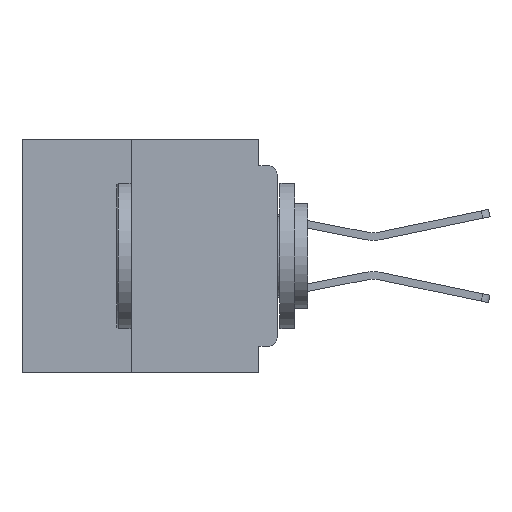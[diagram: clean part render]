
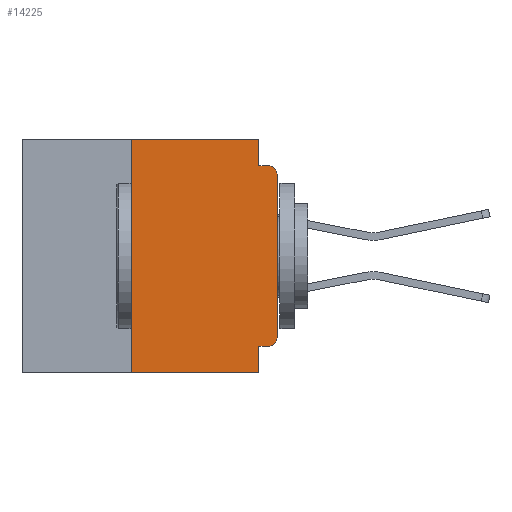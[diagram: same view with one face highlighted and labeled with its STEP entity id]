
A CAD part, left-side view. The second image highlights one B-rep face of the part: STEP entity #14225.
In plain terms, the highlighted planar face has unit normal (-1, 0, 0).
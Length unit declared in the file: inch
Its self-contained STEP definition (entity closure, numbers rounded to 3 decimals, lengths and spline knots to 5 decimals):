
#232 = CARTESIAN_POINT ( 'NONE',  ( 0., 0.25, 0. ) ) ;
#1483 = CARTESIAN_POINT ( 'NONE',  ( 0., 0.031, 0. ) ) ;
#1991 = DIRECTION ( 'NONE',  ( 0., 0., -1. ) ) ;
#2050 = VECTOR ( 'NONE', #49819, 39.37008 ) ;
#2190 = VERTEX_POINT ( 'NONE', #29514 ) ;
#3224 = DIRECTION ( 'NONE',  ( 0., 0., 1. ) ) ;
#3545 = LINE ( 'NONE', #34313, #13835 ) ;
#3659 = EDGE_CURVE ( 'NONE', #49063, #10505, #14028, .T. ) ;
#4939 = EDGE_CURVE ( 'NONE', #13202, #49063, #8471, .T. ) ;
#6959 = DIRECTION ( 'NONE',  ( 0., -1., 0. ) ) ;
#7059 = ORIENTED_EDGE ( 'NONE', *, *, #27937, .F. ) ;
#7067 = AXIS2_PLACEMENT_3D ( 'NONE', #41089, #18066, #44920 ) ;
#7124 = CARTESIAN_POINT ( 'NONE',  ( 0., 0.25, -0.4 ) ) ;
#7233 = CARTESIAN_POINT ( 'NONE',  ( 0., 0., -0.06 ) ) ;
#8471 = LINE ( 'NONE', #38049, #17540 ) ;
#8766 = LINE ( 'NONE', #43683, #28093 ) ;
#8858 = FACE_OUTER_BOUND ( 'NONE', #10433, .T. ) ;
#9204 = VERTEX_POINT ( 'NONE', #7233 ) ;
#9404 = EDGE_CURVE ( 'NONE', #9204, #26934, #10575, .T. ) ;
#10433 = EDGE_LOOP ( 'NONE', ( #49125, #35379, #38479, #33665, #41463, #27238, #47545, #17439, #7059, #19909 ) ) ;
#10505 = VERTEX_POINT ( 'NONE', #47153 ) ;
#10575 = CIRCLE ( 'NONE', #38469, 0.015 ) ;
#13202 = VERTEX_POINT ( 'NONE', #232 ) ;
#13835 = VECTOR ( 'NONE', #49495, 39.37008 ) ;
#14028 = LINE ( 'NONE', #1483, #23120 ) ;
#14183 = PLANE ( 'NONE',  #7067 ) ;
#14225 = ADVANCED_FACE ( 'NONE', ( #8858 ), #14183, .F. ) ;
#15724 = CARTESIAN_POINT ( 'NONE',  ( 0., 0.015, -0.34 ) ) ;
#16689 = CARTESIAN_POINT ( 'NONE',  ( 0., 0.25, -0.4 ) ) ;
#17439 = ORIENTED_EDGE ( 'NONE', *, *, #18331, .F. ) ;
#17540 = VECTOR ( 'NONE', #34218, 39.37008 ) ;
#18066 = DIRECTION ( 'NONE',  ( 1., 0., 0. ) ) ;
#18331 = EDGE_CURVE ( 'NONE', #26631, #31241, #3545, .T. ) ;
#18851 = CARTESIAN_POINT ( 'NONE',  ( 0., 0., -0.045 ) ) ;
#19579 = AXIS2_PLACEMENT_3D ( 'NONE', #15724, #42595, #19598 ) ;
#19598 = DIRECTION ( 'NONE',  ( 0., 0., -1. ) ) ;
#19909 = ORIENTED_EDGE ( 'NONE', *, *, #20971, .T. ) ;
#19921 = DIRECTION ( 'NONE',  ( -1., 0., 0. ) ) ;
#20550 = DIRECTION ( 'NONE',  ( 0., 0., 1. ) ) ;
#20561 = LINE ( 'NONE', #18851, #40963 ) ;
#20971 = EDGE_CURVE ( 'NONE', #44057, #2190, #44777, .T. ) ;
#21524 = VECTOR ( 'NONE', #6959, 39.37008 ) ;
#22809 = CARTESIAN_POINT ( 'NONE',  ( 0., 0.015, -0.045 ) ) ;
#23120 = VECTOR ( 'NONE', #1991, 39.37008 ) ;
#23303 = EDGE_CURVE ( 'NONE', #10505, #26934, #20561, .T. ) ;
#25051 = VECTOR ( 'NONE', #3224, 39.37008 ) ;
#26305 = EDGE_CURVE ( 'NONE', #31709, #31241, #41896, .T. ) ;
#26436 = DIRECTION ( 'NONE',  ( 0., -1., 0. ) ) ;
#26631 = VERTEX_POINT ( 'NONE', #47118 ) ;
#26934 = VERTEX_POINT ( 'NONE', #22809 ) ;
#27238 = ORIENTED_EDGE ( 'NONE', *, *, #33539, .F. ) ;
#27550 = EDGE_CURVE ( 'NONE', #2190, #9204, #8766, .T. ) ;
#27937 = EDGE_CURVE ( 'NONE', #44057, #26631, #40629, .T. ) ;
#28093 = VECTOR ( 'NONE', #20550, 39.37008 ) ;
#29514 = CARTESIAN_POINT ( 'NONE',  ( 0., 0., -0.34 ) ) ;
#29690 = CARTESIAN_POINT ( 'NONE',  ( 0., 0.031, 0. ) ) ;
#31241 = VERTEX_POINT ( 'NONE', #44722 ) ;
#31632 = CARTESIAN_POINT ( 'NONE',  ( 0., 0., -0.355 ) ) ;
#31709 = VERTEX_POINT ( 'NONE', #16689 ) ;
#33539 = EDGE_CURVE ( 'NONE', #31709, #13202, #45430, .T. ) ;
#33665 = ORIENTED_EDGE ( 'NONE', *, *, #3659, .F. ) ;
#34218 = DIRECTION ( 'NONE',  ( 0., -1., 0. ) ) ;
#34313 = CARTESIAN_POINT ( 'NONE',  ( 0., 0.031, -0.4 ) ) ;
#35379 = ORIENTED_EDGE ( 'NONE', *, *, #9404, .T. ) ;
#37777 = CARTESIAN_POINT ( 'NONE',  ( 0., 0.437, -0.4 ) ) ;
#38049 = CARTESIAN_POINT ( 'NONE',  ( 0., 0.437, 0. ) ) ;
#38469 = AXIS2_PLACEMENT_3D ( 'NONE', #42903, #19921, #46754 ) ;
#38479 = ORIENTED_EDGE ( 'NONE', *, *, #23303, .F. ) ;
#40629 = LINE ( 'NONE', #31632, #2050 ) ;
#40963 = VECTOR ( 'NONE', #26436, 39.37008 ) ;
#41089 = CARTESIAN_POINT ( 'NONE',  ( 0., 0.437, 0. ) ) ;
#41463 = ORIENTED_EDGE ( 'NONE', *, *, #4939, .F. ) ;
#41896 = LINE ( 'NONE', #37777, #21524 ) ;
#42595 = DIRECTION ( 'NONE',  ( -1., 0., 0. ) ) ;
#42903 = CARTESIAN_POINT ( 'NONE',  ( 0., 0.015, -0.06 ) ) ;
#43319 = CARTESIAN_POINT ( 'NONE',  ( 0., 0.015, -0.355 ) ) ;
#43683 = CARTESIAN_POINT ( 'NONE',  ( 0., 0., 0. ) ) ;
#44057 = VERTEX_POINT ( 'NONE', #43319 ) ;
#44722 = CARTESIAN_POINT ( 'NONE',  ( 0., 0.031, -0.4 ) ) ;
#44777 = CIRCLE ( 'NONE', #19579, 0.015 ) ;
#44920 = DIRECTION ( 'NONE',  ( 0., 0., -1. ) ) ;
#45430 = LINE ( 'NONE', #7124, #25051 ) ;
#46754 = DIRECTION ( 'NONE',  ( 0., 0., -1. ) ) ;
#47118 = CARTESIAN_POINT ( 'NONE',  ( 0., 0.031, -0.355 ) ) ;
#47153 = CARTESIAN_POINT ( 'NONE',  ( 0., 0.031, -0.045 ) ) ;
#47545 = ORIENTED_EDGE ( 'NONE', *, *, #26305, .T. ) ;
#49063 = VERTEX_POINT ( 'NONE', #29690 ) ;
#49125 = ORIENTED_EDGE ( 'NONE', *, *, #27550, .T. ) ;
#49495 = DIRECTION ( 'NONE',  ( 0., 0., -1. ) ) ;
#49819 = DIRECTION ( 'NONE',  ( 0., 1., 0. ) ) ;
